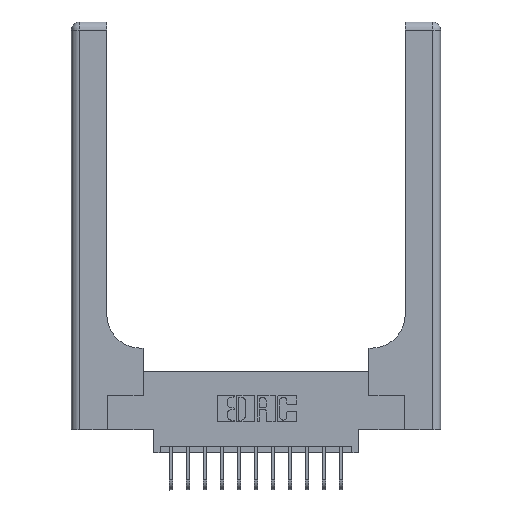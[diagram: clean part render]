
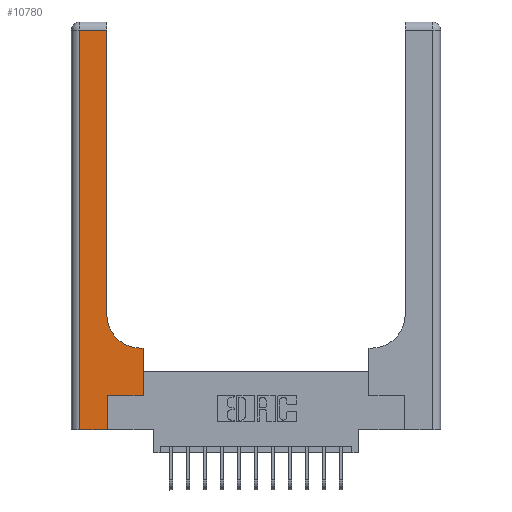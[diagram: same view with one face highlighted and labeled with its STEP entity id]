
A CAD part, top view. The second image highlights one B-rep face of the part: STEP entity #10780.
In plain terms, the highlighted planar face has unit normal (0, 0, 1).
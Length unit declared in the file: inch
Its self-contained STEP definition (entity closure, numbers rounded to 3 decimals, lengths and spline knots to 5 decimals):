
#491 = VERTEX_POINT ( 'NONE', #12235 ) ;
#653 = CARTESIAN_POINT ( 'NONE',  ( 0.06, 0., 0.37 ) ) ;
#852 = DIRECTION ( 'NONE',  ( 0., 0., -1. ) ) ;
#1777 = EDGE_CURVE ( 'NONE', #7441, #491, #10546, .T. ) ;
#2039 = ORIENTED_EDGE ( 'NONE', *, *, #10016, .T. ) ;
#2408 = VECTOR ( 'NONE', #8315, 39.37008 ) ;
#2594 = CARTESIAN_POINT ( 'NONE',  ( 0.528, 0.25, 0.37 ) ) ;
#3125 = CARTESIAN_POINT ( 'NONE',  ( 0.06, 2.94, 0.37 ) ) ;
#3534 = CARTESIAN_POINT ( 'NONE',  ( 0.51, 0.85, 0.37 ) ) ;
#3947 = VECTOR ( 'NONE', #9624, 39.37008 ) ;
#4130 = EDGE_CURVE ( 'NONE', #491, #16354, #13993, .T. ) ;
#4795 = ORIENTED_EDGE ( 'NONE', *, *, #13034, .T. ) ;
#5080 = LINE ( 'NONE', #5720, #5520 ) ;
#5102 = AXIS2_PLACEMENT_3D ( 'NONE', #3534, #852, #6540 ) ;
#5153 = VECTOR ( 'NONE', #8878, 39.37008 ) ;
#5220 = DIRECTION ( 'NONE',  ( -1., 0., 0. ) ) ;
#5309 = LINE ( 'NONE', #8209, #8884 ) ;
#5379 = DIRECTION ( 'NONE',  ( 0., 1., 0. ) ) ;
#5520 = VECTOR ( 'NONE', #5379, 39.37008 ) ;
#5617 = VERTEX_POINT ( 'NONE', #653 ) ;
#5720 = CARTESIAN_POINT ( 'NONE',  ( 0.26, 3., 0.37 ) ) ;
#5750 = ORIENTED_EDGE ( 'NONE', *, *, #11498, .T. ) ;
#6050 = LINE ( 'NONE', #10516, #5153 ) ;
#6540 = DIRECTION ( 'NONE',  ( 1., 0., 0. ) ) ;
#6602 = CARTESIAN_POINT ( 'NONE',  ( 0.265, 0.25, 0.37 ) ) ;
#6834 = DIRECTION ( 'NONE',  ( 1., 0., 0. ) ) ;
#6889 = CARTESIAN_POINT ( 'NONE',  ( 0., 0., 0.37 ) ) ;
#7023 = EDGE_CURVE ( 'NONE', #16354, #16583, #14130, .T. ) ;
#7441 = VERTEX_POINT ( 'NONE', #2594 ) ;
#7526 = CARTESIAN_POINT ( 'NONE',  ( 0., 2.94, 0.37 ) ) ;
#7745 = VERTEX_POINT ( 'NONE', #6602 ) ;
#7842 = PLANE ( 'NONE',  #12667 ) ;
#7949 = DIRECTION ( 'NONE',  ( 0., 1., 0. ) ) ;
#8209 = CARTESIAN_POINT ( 'NONE',  ( 0.265, 0., 0.37 ) ) ;
#8315 = DIRECTION ( 'NONE',  ( 1., 0., 0. ) ) ;
#8538 = FACE_OUTER_BOUND ( 'NONE', #16049, .T. ) ;
#8878 = DIRECTION ( 'NONE',  ( 0., -1., 0. ) ) ;
#8884 = VECTOR ( 'NONE', #7949, 39.37008 ) ;
#8889 = ORIENTED_EDGE ( 'NONE', *, *, #7023, .T. ) ;
#9186 = ORIENTED_EDGE ( 'NONE', *, *, #16186, .T. ) ;
#9418 = CARTESIAN_POINT ( 'NONE',  ( 0., 3., 0.37 ) ) ;
#9624 = DIRECTION ( 'NONE',  ( -1., 0., 0. ) ) ;
#9720 = DIRECTION ( 'NONE',  ( -1., 0., 0. ) ) ;
#9874 = ORIENTED_EDGE ( 'NONE', *, *, #4130, .T. ) ;
#10016 = EDGE_CURVE ( 'NONE', #7745, #7441, #17203, .T. ) ;
#10516 = CARTESIAN_POINT ( 'NONE',  ( 0.06, 3., 0.37 ) ) ;
#10546 = LINE ( 'NONE', #11760, #15865 ) ;
#10780 = ADVANCED_FACE ( 'NONE', ( #8538 ), #7842, .F. ) ;
#10883 = CARTESIAN_POINT ( 'NONE',  ( 0.265, 0., 0.37 ) ) ;
#11498 = EDGE_CURVE ( 'NONE', #12590, #5617, #6050, .T. ) ;
#11760 = CARTESIAN_POINT ( 'NONE',  ( 0.528, 0.25, 0.37 ) ) ;
#12235 = CARTESIAN_POINT ( 'NONE',  ( 0.528, 0.6, 0.37 ) ) ;
#12590 = VERTEX_POINT ( 'NONE', #3125 ) ;
#12667 = AXIS2_PLACEMENT_3D ( 'NONE', #9418, #18228, #9720 ) ;
#13034 = EDGE_CURVE ( 'NONE', #16938, #7745, #5309, .T. ) ;
#13089 = CARTESIAN_POINT ( 'NONE',  ( 0.51, 0.6, 0.37 ) ) ;
#13209 = EDGE_CURVE ( 'NONE', #16583, #13780, #5080, .T. ) ;
#13432 = EDGE_CURVE ( 'NONE', #13780, #12590, #17575, .T. ) ;
#13527 = ORIENTED_EDGE ( 'NONE', *, *, #13432, .T. ) ;
#13780 = VERTEX_POINT ( 'NONE', #14835 ) ;
#13993 = LINE ( 'NONE', #15279, #3947 ) ;
#14130 = CIRCLE ( 'NONE', #5102, 0.25 ) ;
#14335 = CARTESIAN_POINT ( 'NONE',  ( 0.26, 0.85, 0.37 ) ) ;
#14688 = DIRECTION ( 'NONE',  ( 0., 1., 0. ) ) ;
#14835 = CARTESIAN_POINT ( 'NONE',  ( 0.26, 2.94, 0.37 ) ) ;
#14857 = ORIENTED_EDGE ( 'NONE', *, *, #1777, .T. ) ;
#14912 = VECTOR ( 'NONE', #5220, 39.37008 ) ;
#15279 = CARTESIAN_POINT ( 'NONE',  ( 0.26, 0.6, 0.37 ) ) ;
#15664 = VECTOR ( 'NONE', #6834, 39.37008 ) ;
#15865 = VECTOR ( 'NONE', #14688, 39.37008 ) ;
#15925 = ORIENTED_EDGE ( 'NONE', *, *, #13209, .T. ) ;
#16049 = EDGE_LOOP ( 'NONE', ( #15925, #13527, #5750, #9186, #4795, #2039, #14857, #9874, #8889 ) ) ;
#16186 = EDGE_CURVE ( 'NONE', #5617, #16938, #17112, .T. ) ;
#16354 = VERTEX_POINT ( 'NONE', #13089 ) ;
#16583 = VERTEX_POINT ( 'NONE', #14335 ) ;
#16938 = VERTEX_POINT ( 'NONE', #10883 ) ;
#17112 = LINE ( 'NONE', #6889, #2408 ) ;
#17203 = LINE ( 'NONE', #18453, #15664 ) ;
#17575 = LINE ( 'NONE', #7526, #14912 ) ;
#18228 = DIRECTION ( 'NONE',  ( 0., 0., -1. ) ) ;
#18453 = CARTESIAN_POINT ( 'NONE',  ( 0.265, 0.25, 0.37 ) ) ;
